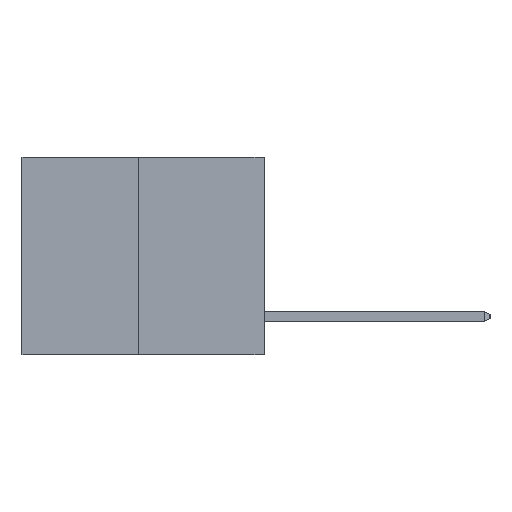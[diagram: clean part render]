
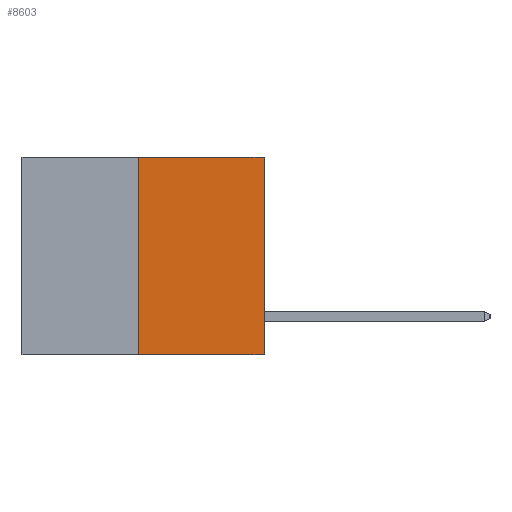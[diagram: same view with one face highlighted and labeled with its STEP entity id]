
A CAD part, left-side view. The second image highlights one B-rep face of the part: STEP entity #8603.
In plain terms, the highlighted planar face has unit normal (-1, 0, 0).
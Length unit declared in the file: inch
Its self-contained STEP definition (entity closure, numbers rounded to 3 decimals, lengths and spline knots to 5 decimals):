
#256 = CARTESIAN_POINT ( 'NONE',  ( 0., 0.6, 0. ) ) ;
#307 = DIRECTION ( 'NONE',  ( 0., 0., -1. ) ) ;
#567 = EDGE_CURVE ( 'NONE', #5429, #4117, #18508, .T. ) ;
#1515 = EDGE_CURVE ( 'NONE', #17713, #5429, #9670, .T. ) ;
#1798 = ORIENTED_EDGE ( 'NONE', *, *, #8508, .F. ) ;
#3307 = CARTESIAN_POINT ( 'NONE',  ( 0., 0., -0.49 ) ) ;
#3343 = LINE ( 'NONE', #19571, #17127 ) ;
#4117 = VERTEX_POINT ( 'NONE', #16914 ) ;
#4160 = LINE ( 'NONE', #13616, #15814 ) ;
#5429 = VERTEX_POINT ( 'NONE', #3307 ) ;
#7683 = DIRECTION ( 'NONE',  ( 0., -1., 0. ) ) ;
#8508 = EDGE_CURVE ( 'NONE', #18994, #4117, #4160, .T. ) ;
#8558 = VECTOR ( 'NONE', #14598, 39.37008 ) ;
#8603 = ADVANCED_FACE ( 'NONE', ( #14129 ), #9589, .F. ) ;
#9118 = CARTESIAN_POINT ( 'NONE',  ( 0., 0.6, -0.49 ) ) ;
#9589 = PLANE ( 'NONE',  #16889 ) ;
#9670 = LINE ( 'NONE', #9118, #15146 ) ;
#10846 = DIRECTION ( 'NONE',  ( 0., -1., 0. ) ) ;
#12340 = ORIENTED_EDGE ( 'NONE', *, *, #16724, .F. ) ;
#13616 = CARTESIAN_POINT ( 'NONE',  ( 0., 0.6, 0. ) ) ;
#13624 = DIRECTION ( 'NONE',  ( 0., 0., 1. ) ) ;
#13966 = EDGE_LOOP ( 'NONE', ( #12340, #14705, #16398, #1798 ) ) ;
#14129 = FACE_OUTER_BOUND ( 'NONE', #13966, .T. ) ;
#14298 = CARTESIAN_POINT ( 'NONE',  ( 0., 0.312, -0.49 ) ) ;
#14598 = DIRECTION ( 'NONE',  ( 0., 0., 1. ) ) ;
#14705 = ORIENTED_EDGE ( 'NONE', *, *, #1515, .T. ) ;
#15146 = VECTOR ( 'NONE', #10846, 39.37008 ) ;
#15394 = CARTESIAN_POINT ( 'NONE',  ( 0., 0.312, 0. ) ) ;
#15814 = VECTOR ( 'NONE', #7683, 39.37008 ) ;
#15949 = CARTESIAN_POINT ( 'NONE',  ( 0., 0., 0. ) ) ;
#16398 = ORIENTED_EDGE ( 'NONE', *, *, #567, .T. ) ;
#16724 = EDGE_CURVE ( 'NONE', #17713, #18994, #3343, .T. ) ;
#16889 = AXIS2_PLACEMENT_3D ( 'NONE', #256, #18407, #307 ) ;
#16914 = CARTESIAN_POINT ( 'NONE',  ( 0., 0., 0. ) ) ;
#17127 = VECTOR ( 'NONE', #13624, 39.37008 ) ;
#17713 = VERTEX_POINT ( 'NONE', #14298 ) ;
#18407 = DIRECTION ( 'NONE',  ( 1., 0., 0. ) ) ;
#18508 = LINE ( 'NONE', #15949, #8558 ) ;
#18994 = VERTEX_POINT ( 'NONE', #15394 ) ;
#19571 = CARTESIAN_POINT ( 'NONE',  ( 0., 0.312, -0.49 ) ) ;
